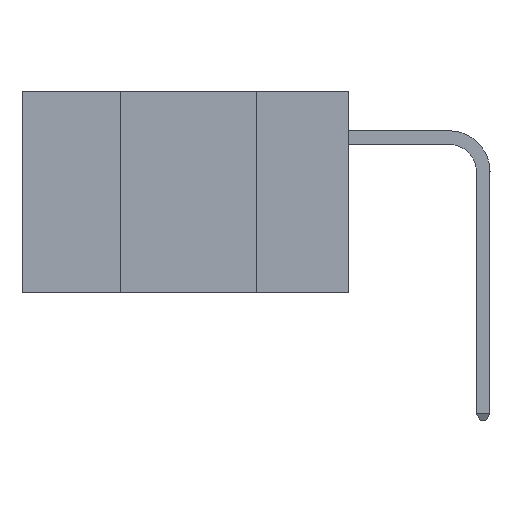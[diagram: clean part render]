
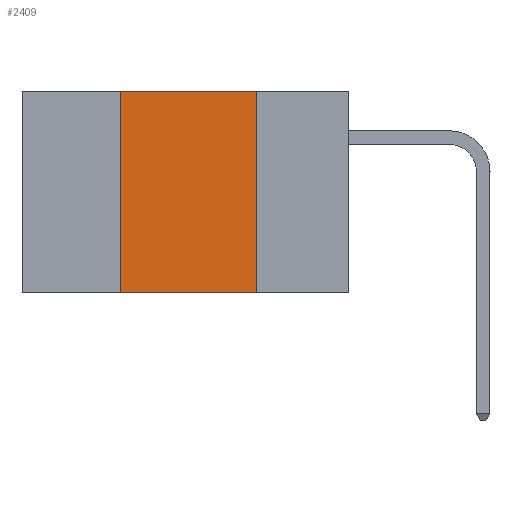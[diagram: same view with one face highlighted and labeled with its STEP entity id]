
A CAD part, left-side view. The second image highlights one B-rep face of the part: STEP entity #2409.
In plain terms, the highlighted planar face has unit normal (-1, 0, 0).
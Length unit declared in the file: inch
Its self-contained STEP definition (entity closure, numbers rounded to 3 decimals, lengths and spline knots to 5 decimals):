
#2246 = LINE ( 'NONE', #11340, #22157 ) ;
#2407 = VECTOR ( 'NONE', #20329, 39.37008 ) ;
#2409 = ADVANCED_FACE ( 'NONE', ( #17130 ), #22486, .F. ) ;
#3652 = EDGE_CURVE ( 'NONE', #5544, #3694, #2246, .T. ) ;
#3694 = VERTEX_POINT ( 'NONE', #11502 ) ;
#3823 = CARTESIAN_POINT ( 'NONE',  ( 0., 0.6, -0.37 ) ) ;
#3899 = CARTESIAN_POINT ( 'NONE',  ( 0., 0.17, -0.37 ) ) ;
#4935 = CARTESIAN_POINT ( 'NONE',  ( 0., 0.17, 0. ) ) ;
#5006 = EDGE_CURVE ( 'NONE', #11577, #17060, #23341, .T. ) ;
#5544 = VERTEX_POINT ( 'NONE', #13416 ) ;
#5763 = DIRECTION ( 'NONE',  ( 0., -1., 0. ) ) ;
#5893 = VECTOR ( 'NONE', #20357, 39.37008 ) ;
#9454 = DIRECTION ( 'NONE',  ( 0., -1., 0. ) ) ;
#11041 = EDGE_LOOP ( 'NONE', ( #14251, #15590, #17604, #21326 ) ) ;
#11340 = CARTESIAN_POINT ( 'NONE',  ( 0., 0.6, 0. ) ) ;
#11502 = CARTESIAN_POINT ( 'NONE',  ( 0., 0.17, 0. ) ) ;
#11577 = VERTEX_POINT ( 'NONE', #12446 ) ;
#12446 = CARTESIAN_POINT ( 'NONE',  ( 0., 0.42, -0.37 ) ) ;
#12896 = DIRECTION ( 'NONE',  ( 0., 0., -1. ) ) ;
#13288 = LINE ( 'NONE', #22169, #2407 ) ;
#13416 = CARTESIAN_POINT ( 'NONE',  ( 0., 0.42, 0. ) ) ;
#14251 = ORIENTED_EDGE ( 'NONE', *, *, #23415, .F. ) ;
#15590 = ORIENTED_EDGE ( 'NONE', *, *, #3652, .F. ) ;
#17060 = VERTEX_POINT ( 'NONE', #3899 ) ;
#17130 = FACE_OUTER_BOUND ( 'NONE', #11041, .T. ) ;
#17604 = ORIENTED_EDGE ( 'NONE', *, *, #19554, .F. ) ;
#17642 = VECTOR ( 'NONE', #5763, 39.37008 ) ;
#18228 = AXIS2_PLACEMENT_3D ( 'NONE', #18621, #24425, #12896 ) ;
#18621 = CARTESIAN_POINT ( 'NONE',  ( 0., 0.6, 0. ) ) ;
#19554 = EDGE_CURVE ( 'NONE', #11577, #5544, #13288, .T. ) ;
#20329 = DIRECTION ( 'NONE',  ( 0., 0., 1. ) ) ;
#20357 = DIRECTION ( 'NONE',  ( 0., 0., -1. ) ) ;
#21272 = LINE ( 'NONE', #4935, #5893 ) ;
#21326 = ORIENTED_EDGE ( 'NONE', *, *, #5006, .T. ) ;
#22157 = VECTOR ( 'NONE', #9454, 39.37008 ) ;
#22169 = CARTESIAN_POINT ( 'NONE',  ( 0., 0.42, 0. ) ) ;
#22486 = PLANE ( 'NONE',  #18228 ) ;
#23341 = LINE ( 'NONE', #3823, #17642 ) ;
#23415 = EDGE_CURVE ( 'NONE', #3694, #17060, #21272, .T. ) ;
#24425 = DIRECTION ( 'NONE',  ( 1., 0., 0. ) ) ;
